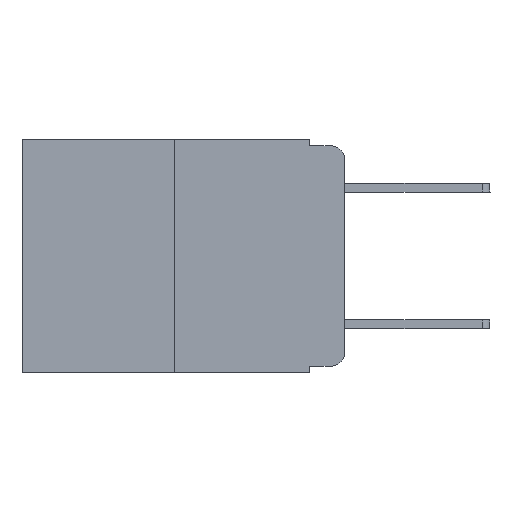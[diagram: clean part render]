
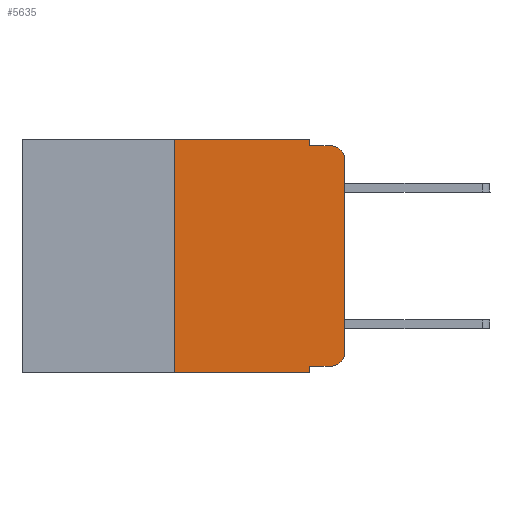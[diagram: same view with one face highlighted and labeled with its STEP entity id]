
A CAD part, left-side view. The second image highlights one B-rep face of the part: STEP entity #5635.
In plain terms, the highlighted planar face has unit normal (-1, 0, 0).
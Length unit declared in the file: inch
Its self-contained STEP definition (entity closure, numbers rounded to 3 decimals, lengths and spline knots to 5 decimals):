
#106 = DIRECTION ( 'NONE',  ( 0., 0., 1. ) ) ;
#132 = VECTOR ( 'NONE', #8594, 39.37008 ) ;
#150 = AXIS2_PLACEMENT_3D ( 'NONE', #4359, #9604, #2029 ) ;
#205 = ORIENTED_EDGE ( 'NONE', *, *, #7846, .T. ) ;
#441 = ORIENTED_EDGE ( 'NONE', *, *, #1208, .T. ) ;
#457 = VERTEX_POINT ( 'NONE', #9490 ) ;
#486 = DIRECTION ( 'NONE',  ( -1., 0., 0. ) ) ;
#540 = CARTESIAN_POINT ( 'NONE',  ( 0., 0.473, 0. ) ) ;
#710 = ORIENTED_EDGE ( 'NONE', *, *, #9356, .T. ) ;
#714 = VECTOR ( 'NONE', #4091, 39.37008 ) ;
#820 = LINE ( 'NONE', #5567, #934 ) ;
#934 = VECTOR ( 'NONE', #5641, 39.37008 ) ;
#941 = EDGE_CURVE ( 'NONE', #5903, #3964, #1549, .T. ) ;
#989 = CARTESIAN_POINT ( 'NONE',  ( 0., 0., 0. ) ) ;
#1081 = CARTESIAN_POINT ( 'NONE',  ( 0., 0.051, -0.01 ) ) ;
#1087 = FACE_OUTER_BOUND ( 'NONE', #3775, .T. ) ;
#1208 = EDGE_CURVE ( 'NONE', #4254, #3358, #3659, .T. ) ;
#1309 = EDGE_CURVE ( 'NONE', #6633, #457, #5186, .T. ) ;
#1549 = LINE ( 'NONE', #5010, #5300 ) ;
#1699 = EDGE_CURVE ( 'NONE', #8089, #6633, #820, .T. ) ;
#2029 = DIRECTION ( 'NONE',  ( 0., 0., -1. ) ) ;
#2035 = VECTOR ( 'NONE', #7086, 39.37008 ) ;
#2038 = DIRECTION ( 'NONE',  ( 0., 0., -1. ) ) ;
#2145 = CARTESIAN_POINT ( 'NONE',  ( 0., 0.051, -0.343 ) ) ;
#2216 = ORIENTED_EDGE ( 'NONE', *, *, #1309, .F. ) ;
#2554 = ORIENTED_EDGE ( 'NONE', *, *, #4163, .F. ) ;
#2686 = ORIENTED_EDGE ( 'NONE', *, *, #941, .T. ) ;
#3012 = AXIS2_PLACEMENT_3D ( 'NONE', #9574, #486, #9505 ) ;
#3045 = CARTESIAN_POINT ( 'NONE',  ( 0., 0.473, 0. ) ) ;
#3106 = ORIENTED_EDGE ( 'NONE', *, *, #5112, .T. ) ;
#3358 = VERTEX_POINT ( 'NONE', #2145 ) ;
#3503 = CARTESIAN_POINT ( 'NONE',  ( 0., 0.051, 0. ) ) ;
#3535 = DIRECTION ( 'NONE',  ( 0., -1., 0. ) ) ;
#3555 = DIRECTION ( 'NONE',  ( 1., 0., 0. ) ) ;
#3659 = LINE ( 'NONE', #7790, #714 ) ;
#3775 = EDGE_LOOP ( 'NONE', ( #205, #710, #2216, #5611, #2554, #7667, #441, #4633, #2686, #3106 ) ) ;
#3806 = AXIS2_PLACEMENT_3D ( 'NONE', #540, #3555, #8930 ) ;
#3901 = VECTOR ( 'NONE', #2038, 39.37008 ) ;
#3964 = VERTEX_POINT ( 'NONE', #6553 ) ;
#4091 = DIRECTION ( 'NONE',  ( 0., -1., 0. ) ) ;
#4163 = EDGE_CURVE ( 'NONE', #6795, #8089, #4515, .T. ) ;
#4254 = VERTEX_POINT ( 'NONE', #9737 ) ;
#4359 = CARTESIAN_POINT ( 'NONE',  ( 0., 0.02, -0.313 ) ) ;
#4515 = LINE ( 'NONE', #3045, #5963 ) ;
#4629 = VERTEX_POINT ( 'NONE', #4777 ) ;
#4633 = ORIENTED_EDGE ( 'NONE', *, *, #7786, .F. ) ;
#4679 = CIRCLE ( 'NONE', #3012, 0.02 ) ;
#4777 = CARTESIAN_POINT ( 'NONE',  ( 0., 0., -0.03 ) ) ;
#4931 = CARTESIAN_POINT ( 'NONE',  ( 0., 0.25, 0. ) ) ;
#5010 = CARTESIAN_POINT ( 'NONE',  ( 0., 0.051, -0.333 ) ) ;
#5112 = EDGE_CURVE ( 'NONE', #3964, #6938, #6535, .T. ) ;
#5179 = VECTOR ( 'NONE', #106, 39.37008 ) ;
#5186 = LINE ( 'NONE', #5562, #132 ) ;
#5300 = VECTOR ( 'NONE', #3535, 39.37008 ) ;
#5336 = DIRECTION ( 'NONE',  ( 0., -1., 0. ) ) ;
#5562 = CARTESIAN_POINT ( 'NONE',  ( 0., 0.051, -0.01 ) ) ;
#5567 = CARTESIAN_POINT ( 'NONE',  ( 0., 0.051, 0. ) ) ;
#5611 = ORIENTED_EDGE ( 'NONE', *, *, #1699, .F. ) ;
#5635 = ADVANCED_FACE ( 'NONE', ( #1087 ), #8902, .F. ) ;
#5641 = DIRECTION ( 'NONE',  ( 0., 0., -1. ) ) ;
#5816 = LINE ( 'NONE', #3503, #3901 ) ;
#5903 = VERTEX_POINT ( 'NONE', #6205 ) ;
#5963 = VECTOR ( 'NONE', #5336, 39.37008 ) ;
#6170 = LINE ( 'NONE', #989, #2035 ) ;
#6205 = CARTESIAN_POINT ( 'NONE',  ( 0., 0.051, -0.333 ) ) ;
#6535 = CIRCLE ( 'NONE', #150, 0.02 ) ;
#6553 = CARTESIAN_POINT ( 'NONE',  ( 0., 0.02, -0.333 ) ) ;
#6633 = VERTEX_POINT ( 'NONE', #1081 ) ;
#6643 = CARTESIAN_POINT ( 'NONE',  ( 0., 0.25, 0. ) ) ;
#6795 = VERTEX_POINT ( 'NONE', #6643 ) ;
#6913 = CARTESIAN_POINT ( 'NONE',  ( 0., 0., -0.313 ) ) ;
#6938 = VERTEX_POINT ( 'NONE', #6913 ) ;
#6978 = LINE ( 'NONE', #4931, #5179 ) ;
#7086 = DIRECTION ( 'NONE',  ( 0., 0., 1. ) ) ;
#7667 = ORIENTED_EDGE ( 'NONE', *, *, #8919, .F. ) ;
#7786 = EDGE_CURVE ( 'NONE', #5903, #3358, #5816, .T. ) ;
#7790 = CARTESIAN_POINT ( 'NONE',  ( 0., 0.473, -0.343 ) ) ;
#7846 = EDGE_CURVE ( 'NONE', #6938, #4629, #6170, .T. ) ;
#8089 = VERTEX_POINT ( 'NONE', #8254 ) ;
#8254 = CARTESIAN_POINT ( 'NONE',  ( 0., 0.051, 0. ) ) ;
#8594 = DIRECTION ( 'NONE',  ( 0., -1., 0. ) ) ;
#8902 = PLANE ( 'NONE',  #3806 ) ;
#8919 = EDGE_CURVE ( 'NONE', #4254, #6795, #6978, .T. ) ;
#8930 = DIRECTION ( 'NONE',  ( 0., 0., -1. ) ) ;
#9356 = EDGE_CURVE ( 'NONE', #4629, #457, #4679, .T. ) ;
#9490 = CARTESIAN_POINT ( 'NONE',  ( 0., 0.02, -0.01 ) ) ;
#9505 = DIRECTION ( 'NONE',  ( 0., 0., -1. ) ) ;
#9574 = CARTESIAN_POINT ( 'NONE',  ( 0., 0.02, -0.03 ) ) ;
#9604 = DIRECTION ( 'NONE',  ( -1., 0., 0. ) ) ;
#9737 = CARTESIAN_POINT ( 'NONE',  ( 0., 0.25, -0.343 ) ) ;
